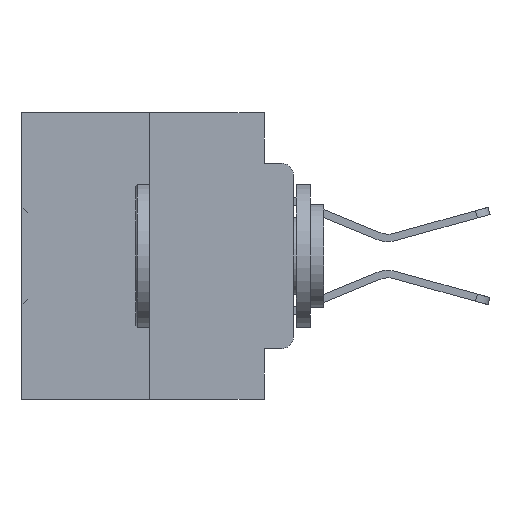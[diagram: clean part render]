
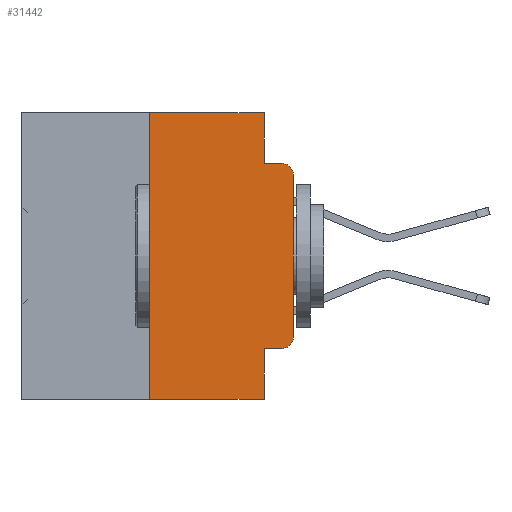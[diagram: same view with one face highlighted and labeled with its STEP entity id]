
A CAD part, left-side view. The second image highlights one B-rep face of the part: STEP entity #31442.
In plain terms, the highlighted planar face has unit normal (-1, 0, 0).
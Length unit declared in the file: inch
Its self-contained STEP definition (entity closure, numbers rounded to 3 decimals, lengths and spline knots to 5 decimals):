
#169 = EDGE_CURVE ( 'NONE', #30539, #29199, #21509, .T. ) ;
#469 = CARTESIAN_POINT ( 'NONE',  ( 0., 0., -0.3915 ) ) ;
#494 = CIRCLE ( 'NONE', #37166, 0.02 ) ;
#928 = LINE ( 'NONE', #18135, #31812 ) ;
#1028 = ORIENTED_EDGE ( 'NONE', *, *, #12155, .F. ) ;
#2186 = EDGE_CURVE ( 'NONE', #30539, #30577, #38073, .T. ) ;
#2196 = DIRECTION ( 'NONE',  ( 0., -1., 0. ) ) ;
#2221 = AXIS2_PLACEMENT_3D ( 'NONE', #28528, #10539, #31522 ) ;
#2606 = CARTESIAN_POINT ( 'NONE',  ( 0., 0.02, -0.1085 ) ) ;
#3162 = LINE ( 'NONE', #5208, #33973 ) ;
#3720 = VERTEX_POINT ( 'NONE', #10126 ) ;
#3841 = ORIENTED_EDGE ( 'NONE', *, *, #4180, .F. ) ;
#3964 = VERTEX_POINT ( 'NONE', #25740 ) ;
#4180 = EDGE_CURVE ( 'NONE', #34505, #13170, #38214, .T. ) ;
#4294 = CARTESIAN_POINT ( 'NONE',  ( 0., 0.25, 0. ) ) ;
#5208 = CARTESIAN_POINT ( 'NONE',  ( 0., 0., 0. ) ) ;
#5266 = EDGE_LOOP ( 'NONE', ( #7027, #23989, #1028, #24930, #18828, #3841, #20712, #36463, #22601, #16486 ) ) ;
#5593 = DIRECTION ( 'NONE',  ( 0., 0., -1. ) ) ;
#5596 = VECTOR ( 'NONE', #19386, 39.37008 ) ;
#6338 = CARTESIAN_POINT ( 'NONE',  ( 0., 0.473, 0. ) ) ;
#7027 = ORIENTED_EDGE ( 'NONE', *, *, #18211, .T. ) ;
#9142 = DIRECTION ( 'NONE',  ( 0., -1., 0. ) ) ;
#10057 = CARTESIAN_POINT ( 'NONE',  ( 0., 0.051, -0.4115 ) ) ;
#10120 = EDGE_CURVE ( 'NONE', #3720, #15591, #10335, .T. ) ;
#10126 = CARTESIAN_POINT ( 'NONE',  ( 0., 0.051, 0. ) ) ;
#10184 = CARTESIAN_POINT ( 'NONE',  ( 0., 0.051, -0.5 ) ) ;
#10335 = LINE ( 'NONE', #11162, #25392 ) ;
#10530 = DIRECTION ( 'NONE',  ( 0., 0., 1. ) ) ;
#10539 = DIRECTION ( 'NONE',  ( 1., 0., 0. ) ) ;
#11162 = CARTESIAN_POINT ( 'NONE',  ( 0., 0.051, 0. ) ) ;
#12023 = DIRECTION ( 'NONE',  ( -1., 0., 0. ) ) ;
#12155 = EDGE_CURVE ( 'NONE', #15591, #3964, #27548, .T. ) ;
#12401 = VERTEX_POINT ( 'NONE', #469 ) ;
#12806 = VERTEX_POINT ( 'NONE', #17181 ) ;
#13170 = VERTEX_POINT ( 'NONE', #36772 ) ;
#14083 = DIRECTION ( 'NONE',  ( 0., 0., 1. ) ) ;
#14194 = EDGE_CURVE ( 'NONE', #12806, #3964, #20457, .T. ) ;
#15192 = LINE ( 'NONE', #6338, #22216 ) ;
#15591 = VERTEX_POINT ( 'NONE', #27365 ) ;
#16486 = ORIENTED_EDGE ( 'NONE', *, *, #32938, .T. ) ;
#17181 = CARTESIAN_POINT ( 'NONE',  ( 0., 0., -0.1085 ) ) ;
#17235 = DIRECTION ( 'NONE',  ( 0., 0., -1. ) ) ;
#17340 = CARTESIAN_POINT ( 'NONE',  ( 0., 0.051, 0. ) ) ;
#18135 = CARTESIAN_POINT ( 'NONE',  ( 0., 0.473, -0.5 ) ) ;
#18211 = EDGE_CURVE ( 'NONE', #12401, #12806, #3162, .T. ) ;
#18828 = ORIENTED_EDGE ( 'NONE', *, *, #29774, .F. ) ;
#19386 = DIRECTION ( 'NONE',  ( 0., -1., 0. ) ) ;
#20457 = CIRCLE ( 'NONE', #25379, 0.02 ) ;
#20712 = ORIENTED_EDGE ( 'NONE', *, *, #24026, .T. ) ;
#21509 = LINE ( 'NONE', #27390, #5596 ) ;
#22133 = CARTESIAN_POINT ( 'NONE',  ( 0., 0.25, -0.5 ) ) ;
#22216 = VECTOR ( 'NONE', #30326, 39.37008 ) ;
#22534 = PLANE ( 'NONE',  #2221 ) ;
#22601 = ORIENTED_EDGE ( 'NONE', *, *, #169, .T. ) ;
#23565 = DIRECTION ( 'NONE',  ( -1., 0., 0. ) ) ;
#23989 = ORIENTED_EDGE ( 'NONE', *, *, #14194, .T. ) ;
#24026 = EDGE_CURVE ( 'NONE', #34505, #30577, #928, .T. ) ;
#24930 = ORIENTED_EDGE ( 'NONE', *, *, #10120, .F. ) ;
#25379 = AXIS2_PLACEMENT_3D ( 'NONE', #2606, #23565, #5593 ) ;
#25387 = DIRECTION ( 'NONE',  ( 0., 0., -1. ) ) ;
#25392 = VECTOR ( 'NONE', #17235, 39.37008 ) ;
#25740 = CARTESIAN_POINT ( 'NONE',  ( 0., 0.02, -0.0885 ) ) ;
#26630 = VECTOR ( 'NONE', #2196, 39.37008 ) ;
#27365 = CARTESIAN_POINT ( 'NONE',  ( 0., 0.051, -0.0885 ) ) ;
#27390 = CARTESIAN_POINT ( 'NONE',  ( 0., 0.051, -0.4115 ) ) ;
#27548 = LINE ( 'NONE', #32006, #26630 ) ;
#27621 = CARTESIAN_POINT ( 'NONE',  ( 0., 0.02, -0.4115 ) ) ;
#28528 = CARTESIAN_POINT ( 'NONE',  ( 0., 0.473, 0. ) ) ;
#28591 = VECTOR ( 'NONE', #10530, 39.37008 ) ;
#29199 = VERTEX_POINT ( 'NONE', #27621 ) ;
#29562 = FACE_OUTER_BOUND ( 'NONE', #5266, .T. ) ;
#29774 = EDGE_CURVE ( 'NONE', #13170, #3720, #15192, .T. ) ;
#29978 = CARTESIAN_POINT ( 'NONE',  ( 0., 0.02, -0.3915 ) ) ;
#30308 = VECTOR ( 'NONE', #25387, 39.37008 ) ;
#30326 = DIRECTION ( 'NONE',  ( 0., -1., 0. ) ) ;
#30539 = VERTEX_POINT ( 'NONE', #10057 ) ;
#30577 = VERTEX_POINT ( 'NONE', #10184 ) ;
#31442 = ADVANCED_FACE ( 'NONE', ( #29562 ), #22534, .F. ) ;
#31522 = DIRECTION ( 'NONE',  ( 0., 0., -1. ) ) ;
#31812 = VECTOR ( 'NONE', #9142, 39.37008 ) ;
#32006 = CARTESIAN_POINT ( 'NONE',  ( 0., 0.051, -0.0885 ) ) ;
#32937 = DIRECTION ( 'NONE',  ( 0., 0., -1. ) ) ;
#32938 = EDGE_CURVE ( 'NONE', #29199, #12401, #494, .T. ) ;
#33973 = VECTOR ( 'NONE', #14083, 39.37008 ) ;
#34505 = VERTEX_POINT ( 'NONE', #22133 ) ;
#36463 = ORIENTED_EDGE ( 'NONE', *, *, #2186, .F. ) ;
#36772 = CARTESIAN_POINT ( 'NONE',  ( 0., 0.25, 0. ) ) ;
#37166 = AXIS2_PLACEMENT_3D ( 'NONE', #29978, #12023, #32937 ) ;
#38073 = LINE ( 'NONE', #17340, #30308 ) ;
#38214 = LINE ( 'NONE', #4294, #28591 ) ;
